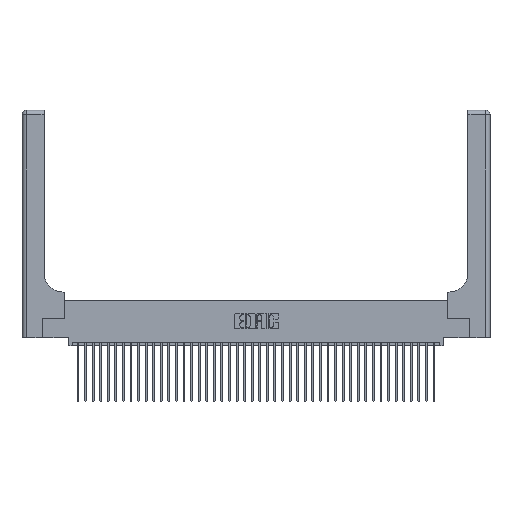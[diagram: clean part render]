
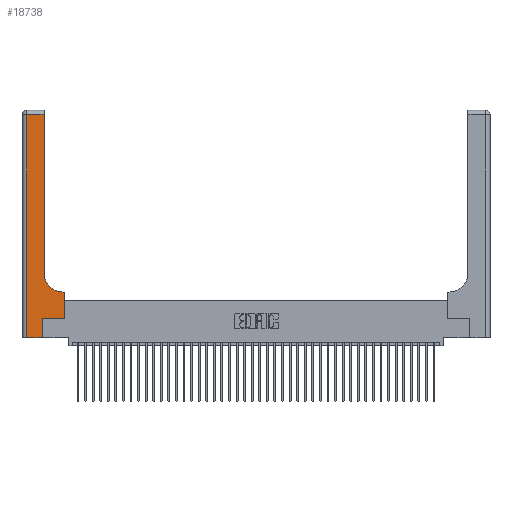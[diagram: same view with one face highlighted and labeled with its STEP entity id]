
A CAD part, top view. The second image highlights one B-rep face of the part: STEP entity #18738.
In plain terms, the highlighted planar face has unit normal (0, 0, 1).
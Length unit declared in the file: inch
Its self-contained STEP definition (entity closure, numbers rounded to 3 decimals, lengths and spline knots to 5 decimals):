
#652 = DIRECTION ( 'NONE',  ( 0., 0., -1. ) ) ;
#1981 = CARTESIAN_POINT ( 'NONE',  ( 0., 2.94, 0.37 ) ) ;
#2483 = CARTESIAN_POINT ( 'NONE',  ( 0.269, 0., 0.37 ) ) ;
#2487 = VERTEX_POINT ( 'NONE', #18494 ) ;
#2732 = ORIENTED_EDGE ( 'NONE', *, *, #12052, .T. ) ;
#2976 = AXIS2_PLACEMENT_3D ( 'NONE', #32279, #652, #26701 ) ;
#3712 = VERTEX_POINT ( 'NONE', #38360 ) ;
#4052 = VERTEX_POINT ( 'NONE', #14517 ) ;
#4198 = CARTESIAN_POINT ( 'NONE',  ( 0., 0., 0.37 ) ) ;
#4654 = LINE ( 'NONE', #14192, #28574 ) ;
#5216 = AXIS2_PLACEMENT_3D ( 'NONE', #35292, #9415, #19222 ) ;
#6117 = DIRECTION ( 'NONE',  ( 0., 1., 0. ) ) ;
#6255 = ORIENTED_EDGE ( 'NONE', *, *, #35002, .T. ) ;
#7559 = VECTOR ( 'NONE', #6117, 39.37008 ) ;
#7707 = ORIENTED_EDGE ( 'NONE', *, *, #25519, .T. ) ;
#8954 = VERTEX_POINT ( 'NONE', #14770 ) ;
#9415 = DIRECTION ( 'NONE',  ( 0., 0., -1. ) ) ;
#9571 = VERTEX_POINT ( 'NONE', #30021 ) ;
#10105 = EDGE_CURVE ( 'NONE', #16068, #3712, #16329, .T. ) ;
#10268 = ORIENTED_EDGE ( 'NONE', *, *, #10105, .T. ) ;
#10742 = VECTOR ( 'NONE', #40533, 39.37008 ) ;
#11669 = DIRECTION ( 'NONE',  ( 0., 1., 0. ) ) ;
#12052 = EDGE_CURVE ( 'NONE', #2487, #36576, #35052, .T. ) ;
#13021 = ORIENTED_EDGE ( 'NONE', *, *, #20534, .T. ) ;
#13676 = VECTOR ( 'NONE', #30080, 39.37008 ) ;
#14192 = CARTESIAN_POINT ( 'NONE',  ( 0.06, 3., 0.37 ) ) ;
#14517 = CARTESIAN_POINT ( 'NONE',  ( 0.06, 0., 0.37 ) ) ;
#14770 = CARTESIAN_POINT ( 'NONE',  ( 0.5415, 0.6, 0.37 ) ) ;
#14857 = ORIENTED_EDGE ( 'NONE', *, *, #41014, .T. ) ;
#15215 = VECTOR ( 'NONE', #22288, 39.37008 ) ;
#15632 = PLANE ( 'NONE',  #2976 ) ;
#16068 = VERTEX_POINT ( 'NONE', #33995 ) ;
#16329 = LINE ( 'NONE', #17163, #10742 ) ;
#16734 = ORIENTED_EDGE ( 'NONE', *, *, #23539, .T. ) ;
#17163 = CARTESIAN_POINT ( 'NONE',  ( 0.269, 0.25, 0.37 ) ) ;
#17423 = CARTESIAN_POINT ( 'NONE',  ( 0.2915, 2.94, 0.37 ) ) ;
#17771 = CARTESIAN_POINT ( 'NONE',  ( 0.5585, 0.25, 0.37 ) ) ;
#18349 = FACE_OUTER_BOUND ( 'NONE', #40164, .T. ) ;
#18494 = CARTESIAN_POINT ( 'NONE',  ( 0.2915, 0.85, 0.37 ) ) ;
#18738 = ADVANCED_FACE ( 'NONE', ( #18349 ), #15632, .F. ) ;
#19222 = DIRECTION ( 'NONE',  ( 1., 0., 0. ) ) ;
#19875 = VECTOR ( 'NONE', #11669, 39.37008 ) ;
#20129 = VECTOR ( 'NONE', #24753, 39.37008 ) ;
#20352 = LINE ( 'NONE', #17771, #19875 ) ;
#20534 = EDGE_CURVE ( 'NONE', #4052, #25298, #23875, .T. ) ;
#22288 = DIRECTION ( 'NONE',  ( 0., 1., 0. ) ) ;
#23539 = EDGE_CURVE ( 'NONE', #36576, #9571, #29271, .T. ) ;
#23875 = LINE ( 'NONE', #4198, #13676 ) ;
#24020 = LINE ( 'NONE', #36532, #29131 ) ;
#24753 = DIRECTION ( 'NONE',  ( -1., 0., 0. ) ) ;
#25298 = VERTEX_POINT ( 'NONE', #26909 ) ;
#25519 = EDGE_CURVE ( 'NONE', #34531, #8954, #24020, .T. ) ;
#26701 = DIRECTION ( 'NONE',  ( -1., 0., 0. ) ) ;
#26909 = CARTESIAN_POINT ( 'NONE',  ( 0.269, 0., 0.37 ) ) ;
#27433 = EDGE_CURVE ( 'NONE', #3712, #34531, #20352, .T. ) ;
#27940 = LINE ( 'NONE', #2483, #15215 ) ;
#28317 = CARTESIAN_POINT ( 'NONE',  ( 0.5585, 0.6, 0.37 ) ) ;
#28574 = VECTOR ( 'NONE', #33273, 39.37008 ) ;
#29131 = VECTOR ( 'NONE', #39975, 39.37008 ) ;
#29271 = LINE ( 'NONE', #1981, #20129 ) ;
#30021 = CARTESIAN_POINT ( 'NONE',  ( 0.06, 2.94, 0.37 ) ) ;
#30080 = DIRECTION ( 'NONE',  ( 1., 0., 0. ) ) ;
#30151 = CARTESIAN_POINT ( 'NONE',  ( 0.2915, 3., 0.37 ) ) ;
#32279 = CARTESIAN_POINT ( 'NONE',  ( 0., 3., 0.37 ) ) ;
#32961 = ORIENTED_EDGE ( 'NONE', *, *, #27433, .T. ) ;
#33273 = DIRECTION ( 'NONE',  ( 0., -1., 0. ) ) ;
#33742 = CIRCLE ( 'NONE', #5216, 0.25 ) ;
#33995 = CARTESIAN_POINT ( 'NONE',  ( 0.269, 0.25, 0.37 ) ) ;
#34531 = VERTEX_POINT ( 'NONE', #28317 ) ;
#35002 = EDGE_CURVE ( 'NONE', #9571, #4052, #4654, .T. ) ;
#35052 = LINE ( 'NONE', #30151, #7559 ) ;
#35292 = CARTESIAN_POINT ( 'NONE',  ( 0.5415, 0.85, 0.37 ) ) ;
#36532 = CARTESIAN_POINT ( 'NONE',  ( 0.2915, 0.6, 0.37 ) ) ;
#36576 = VERTEX_POINT ( 'NONE', #17423 ) ;
#38360 = CARTESIAN_POINT ( 'NONE',  ( 0.5585, 0.25, 0.37 ) ) ;
#39975 = DIRECTION ( 'NONE',  ( -1., 0., 0. ) ) ;
#40164 = EDGE_LOOP ( 'NONE', ( #2732, #16734, #6255, #13021, #41709, #10268, #32961, #7707, #14857 ) ) ;
#40533 = DIRECTION ( 'NONE',  ( 1., 0., 0. ) ) ;
#41014 = EDGE_CURVE ( 'NONE', #8954, #2487, #33742, .T. ) ;
#41583 = EDGE_CURVE ( 'NONE', #25298, #16068, #27940, .T. ) ;
#41709 = ORIENTED_EDGE ( 'NONE', *, *, #41583, .T. ) ;
